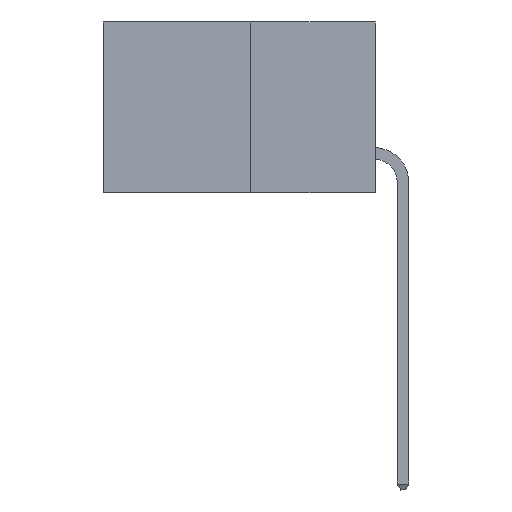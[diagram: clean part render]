
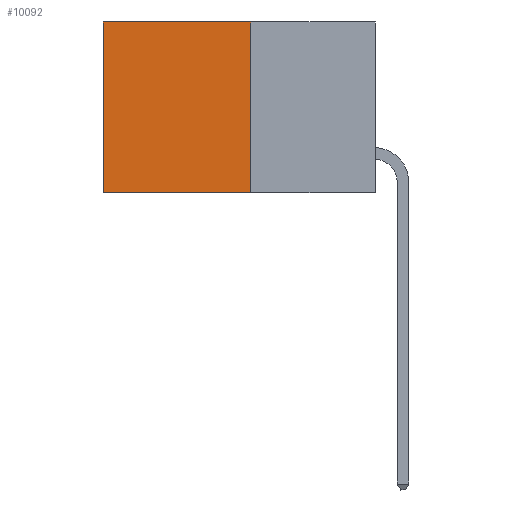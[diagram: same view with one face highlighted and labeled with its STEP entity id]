
A CAD part, left-side view. The second image highlights one B-rep face of the part: STEP entity #10092.
In plain terms, the highlighted planar face has unit normal (-1, 0, 0).
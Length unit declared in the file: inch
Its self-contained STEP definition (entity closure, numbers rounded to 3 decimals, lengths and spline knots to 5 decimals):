
#94 = CARTESIAN_POINT ( 'NONE',  ( 0.277, 0.59, 0. ) ) ;
#279 = LINE ( 'NONE', #1034, #9933 ) ;
#321 = EDGE_CURVE ( 'NONE', #5183, #745, #11469, .T. ) ;
#465 = CARTESIAN_POINT ( 'NONE',  ( 0.277, 0.27, -0.37 ) ) ;
#745 = VERTEX_POINT ( 'NONE', #8889 ) ;
#1011 = PLANE ( 'NONE',  #3194 ) ;
#1034 = CARTESIAN_POINT ( 'NONE',  ( 0.277, 0.27, -0.37 ) ) ;
#1061 = EDGE_CURVE ( 'NONE', #8628, #8591, #10238, .T. ) ;
#1733 = VECTOR ( 'NONE', #8363, 39.37008 ) ;
#2015 = FACE_OUTER_BOUND ( 'NONE', #8104, .T. ) ;
#3194 = AXIS2_PLACEMENT_3D ( 'NONE', #11057, #3545, #12320 ) ;
#3545 = DIRECTION ( 'NONE',  ( 1., 0., 0. ) ) ;
#5183 = VERTEX_POINT ( 'NONE', #7574 ) ;
#5249 = ORIENTED_EDGE ( 'NONE', *, *, #1061, .T. ) ;
#6288 = ORIENTED_EDGE ( 'NONE', *, *, #15972, .F. ) ;
#6687 = ORIENTED_EDGE ( 'NONE', *, *, #15215, .T. ) ;
#7060 = CARTESIAN_POINT ( 'NONE',  ( 0.277, 0.27, 0. ) ) ;
#7574 = CARTESIAN_POINT ( 'NONE',  ( 0.277, 0.27, 0. ) ) ;
#8104 = EDGE_LOOP ( 'NONE', ( #5249, #6288, #15268, #6687 ) ) ;
#8363 = DIRECTION ( 'NONE',  ( 0., 1., 0. ) ) ;
#8364 = LINE ( 'NONE', #7060, #1733 ) ;
#8425 = DIRECTION ( 'NONE',  ( 0., 0., -1. ) ) ;
#8515 = DIRECTION ( 'NONE',  ( 0., 1., 0. ) ) ;
#8591 = VERTEX_POINT ( 'NONE', #15096 ) ;
#8628 = VERTEX_POINT ( 'NONE', #94 ) ;
#8889 = CARTESIAN_POINT ( 'NONE',  ( 0.277, 0.27, -0.37 ) ) ;
#9933 = VECTOR ( 'NONE', #8515, 39.37008 ) ;
#10092 = ADVANCED_FACE ( 'NONE', ( #2015 ), #1011, .F. ) ;
#10238 = LINE ( 'NONE', #15430, #13584 ) ;
#11057 = CARTESIAN_POINT ( 'NONE',  ( 0.277, 0.27, -0.37 ) ) ;
#11469 = LINE ( 'NONE', #465, #14375 ) ;
#12320 = DIRECTION ( 'NONE',  ( 0., 0., -1. ) ) ;
#13584 = VECTOR ( 'NONE', #14856, 39.37008 ) ;
#14375 = VECTOR ( 'NONE', #8425, 39.37008 ) ;
#14856 = DIRECTION ( 'NONE',  ( 0., 0., -1. ) ) ;
#15096 = CARTESIAN_POINT ( 'NONE',  ( 0.277, 0.59, -0.37 ) ) ;
#15215 = EDGE_CURVE ( 'NONE', #5183, #8628, #8364, .T. ) ;
#15268 = ORIENTED_EDGE ( 'NONE', *, *, #321, .F. ) ;
#15430 = CARTESIAN_POINT ( 'NONE',  ( 0.277, 0.59, -0.37 ) ) ;
#15972 = EDGE_CURVE ( 'NONE', #745, #8591, #279, .T. ) ;
